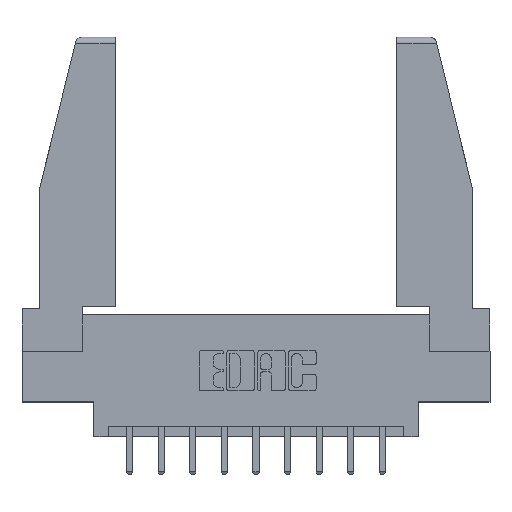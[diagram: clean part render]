
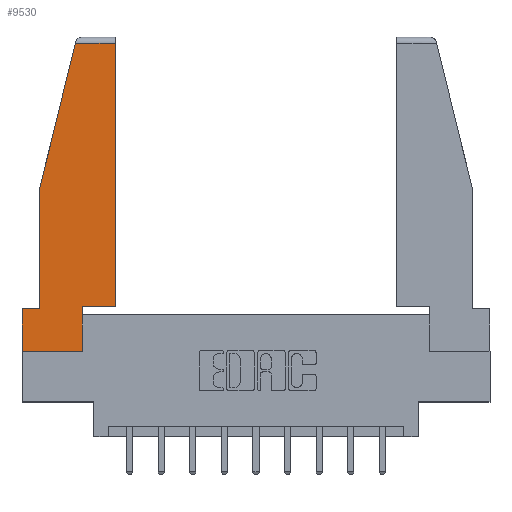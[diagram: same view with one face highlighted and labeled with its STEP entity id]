
A CAD part, top view. The second image highlights one B-rep face of the part: STEP entity #9530.
In plain terms, the highlighted planar face has unit normal (0, 0, 1).
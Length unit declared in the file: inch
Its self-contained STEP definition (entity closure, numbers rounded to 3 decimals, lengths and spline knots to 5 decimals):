
#599 = LINE ( 'NONE', #7485, #6048 ) ;
#632 = LINE ( 'NONE', #3141, #11738 ) ;
#886 = ORIENTED_EDGE ( 'NONE', *, *, #2664, .T. ) ;
#963 = CARTESIAN_POINT ( 'NONE',  ( 0., 0., 0. ) ) ;
#1151 = VERTEX_POINT ( 'NONE', #7182 ) ;
#1693 = ORIENTED_EDGE ( 'NONE', *, *, #10369, .T. ) ;
#2319 = CARTESIAN_POINT ( 'NONE',  ( 0., 0.21, 0. ) ) ;
#2331 = LINE ( 'NONE', #963, #5567 ) ;
#2338 = CARTESIAN_POINT ( 'NONE',  ( 0.2636, 1.52, 0. ) ) ;
#2345 = ORIENTED_EDGE ( 'NONE', *, *, #7539, .T. ) ;
#2501 = CARTESIAN_POINT ( 'NONE',  ( 0., 0.21, 0. ) ) ;
#2664 = EDGE_CURVE ( 'NONE', #3824, #9317, #599, .T. ) ;
#2733 = LINE ( 'NONE', #4475, #7913 ) ;
#3004 = VERTEX_POINT ( 'NONE', #5053 ) ;
#3141 = CARTESIAN_POINT ( 'NONE',  ( 0.297, 0., 0. ) ) ;
#3367 = EDGE_CURVE ( 'NONE', #7564, #3004, #7673, .T. ) ;
#3384 = ORIENTED_EDGE ( 'NONE', *, *, #9547, .T. ) ;
#3464 = VECTOR ( 'NONE', #13909, 39.37008 ) ;
#3678 = CARTESIAN_POINT ( 'NONE',  ( 0.461, 0.223, 0. ) ) ;
#3699 = ORIENTED_EDGE ( 'NONE', *, *, #5923, .T. ) ;
#3819 = CARTESIAN_POINT ( 'NONE',  ( 0., 0.21, 0. ) ) ;
#3824 = VERTEX_POINT ( 'NONE', #12988 ) ;
#3905 = DIRECTION ( 'NONE',  ( 1., 0., 0. ) ) ;
#4475 = CARTESIAN_POINT ( 'NONE',  ( 0., 1.52, 0. ) ) ;
#4582 = CARTESIAN_POINT ( 'NONE',  ( 0.461, 1.52, 0. ) ) ;
#4804 = ORIENTED_EDGE ( 'NONE', *, *, #3367, .T. ) ;
#5027 = CARTESIAN_POINT ( 'NONE',  ( 0.297, 0., 0. ) ) ;
#5053 = CARTESIAN_POINT ( 'NONE',  ( 0.086, 0.8, 0. ) ) ;
#5086 = LINE ( 'NONE', #3678, #11765 ) ;
#5281 = CARTESIAN_POINT ( 'NONE',  ( 0., 0., 0. ) ) ;
#5567 = VECTOR ( 'NONE', #10732, 39.37008 ) ;
#5923 = EDGE_CURVE ( 'NONE', #11794, #3824, #632, .T. ) ;
#6043 = CARTESIAN_POINT ( 'NONE',  ( 0., 0., 0. ) ) ;
#6048 = VECTOR ( 'NONE', #9933, 39.37008 ) ;
#6260 = EDGE_CURVE ( 'NONE', #11692, #11794, #2331, .T. ) ;
#6267 = AXIS2_PLACEMENT_3D ( 'NONE', #6043, #8208, #3905 ) ;
#6354 = CARTESIAN_POINT ( 'NONE',  ( 0.086, 0.8, 0. ) ) ;
#6523 = ORIENTED_EDGE ( 'NONE', *, *, #12342, .T. ) ;
#7182 = CARTESIAN_POINT ( 'NONE',  ( 0.086, 0.21, 0. ) ) ;
#7286 = VECTOR ( 'NONE', #9976, 39.37008 ) ;
#7294 = VERTEX_POINT ( 'NONE', #3819 ) ;
#7485 = CARTESIAN_POINT ( 'NONE',  ( 0.297, 0.223, 0. ) ) ;
#7539 = EDGE_CURVE ( 'NONE', #3004, #1151, #8813, .T. ) ;
#7564 = VERTEX_POINT ( 'NONE', #2338 ) ;
#7673 = LINE ( 'NONE', #8010, #12198 ) ;
#7701 = EDGE_LOOP ( 'NONE', ( #3384, #8531, #4804, #2345, #1693, #6523, #13694, #3699, #886 ) ) ;
#7913 = VECTOR ( 'NONE', #13234, 39.37008 ) ;
#8010 = CARTESIAN_POINT ( 'NONE',  ( 0.271, 1.55, 0. ) ) ;
#8208 = DIRECTION ( 'NONE',  ( 0., 0., 1. ) ) ;
#8531 = ORIENTED_EDGE ( 'NONE', *, *, #9527, .T. ) ;
#8555 = DIRECTION ( 'NONE',  ( 0., 1., 0. ) ) ;
#8813 = LINE ( 'NONE', #6354, #3464 ) ;
#9243 = FACE_OUTER_BOUND ( 'NONE', #7701, .T. ) ;
#9317 = VERTEX_POINT ( 'NONE', #10778 ) ;
#9351 = DIRECTION ( 'NONE',  ( 0., 1., 0. ) ) ;
#9527 = EDGE_CURVE ( 'NONE', #11386, #7564, #2733, .T. ) ;
#9530 = ADVANCED_FACE ( 'NONE', ( #9243 ), #13382, .T. ) ;
#9547 = EDGE_CURVE ( 'NONE', #9317, #11386, #5086, .T. ) ;
#9834 = DIRECTION ( 'NONE',  ( -1., 0., 0. ) ) ;
#9933 = DIRECTION ( 'NONE',  ( 1., 0., 0. ) ) ;
#9950 = DIRECTION ( 'NONE',  ( -0.239, -0.971, 0. ) ) ;
#9976 = DIRECTION ( 'NONE',  ( 0., -1., 0. ) ) ;
#10167 = VECTOR ( 'NONE', #9834, 39.37008 ) ;
#10369 = EDGE_CURVE ( 'NONE', #1151, #7294, #11686, .T. ) ;
#10449 = LINE ( 'NONE', #2501, #7286 ) ;
#10732 = DIRECTION ( 'NONE',  ( 1., 0., 0. ) ) ;
#10778 = CARTESIAN_POINT ( 'NONE',  ( 0.461, 0.223, 0. ) ) ;
#11386 = VERTEX_POINT ( 'NONE', #4582 ) ;
#11686 = LINE ( 'NONE', #2319, #10167 ) ;
#11692 = VERTEX_POINT ( 'NONE', #5281 ) ;
#11738 = VECTOR ( 'NONE', #8555, 39.37008 ) ;
#11765 = VECTOR ( 'NONE', #9351, 39.37008 ) ;
#11794 = VERTEX_POINT ( 'NONE', #5027 ) ;
#12198 = VECTOR ( 'NONE', #9950, 39.37008 ) ;
#12342 = EDGE_CURVE ( 'NONE', #7294, #11692, #10449, .T. ) ;
#12988 = CARTESIAN_POINT ( 'NONE',  ( 0.297, 0.223, 0. ) ) ;
#13234 = DIRECTION ( 'NONE',  ( -1., 0., 0. ) ) ;
#13382 = PLANE ( 'NONE',  #6267 ) ;
#13694 = ORIENTED_EDGE ( 'NONE', *, *, #6260, .T. ) ;
#13909 = DIRECTION ( 'NONE',  ( 0., -1., 0. ) ) ;
